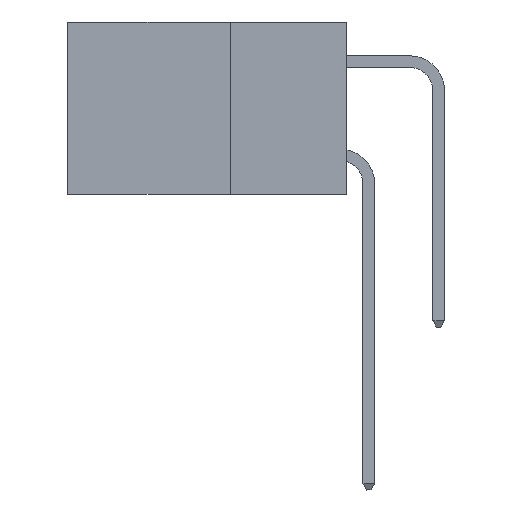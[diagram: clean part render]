
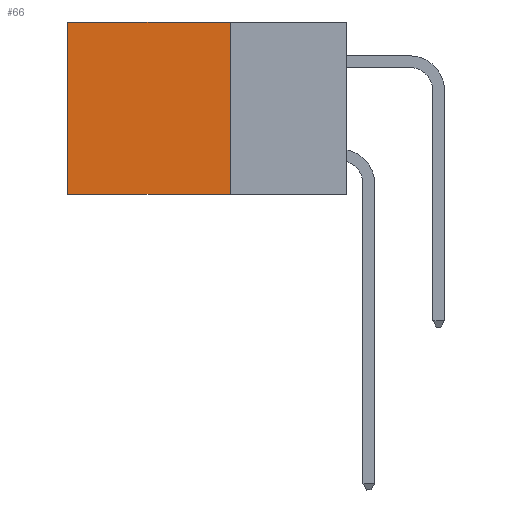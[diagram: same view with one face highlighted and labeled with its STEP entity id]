
A CAD part, left-side view. The second image highlights one B-rep face of the part: STEP entity #66.
In plain terms, the highlighted planar face has unit normal (-1, 0, 0).
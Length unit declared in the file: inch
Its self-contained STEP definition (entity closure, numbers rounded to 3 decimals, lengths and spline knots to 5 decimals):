
#66 = ADVANCED_FACE ( 'NONE', ( #22812 ), #25217, .F. ) ;
#1193 = ORIENTED_EDGE ( 'NONE', *, *, #30866, .T. ) ;
#2243 = CARTESIAN_POINT ( 'NONE',  ( 0.2875, 0.6, -0.37 ) ) ;
#3347 = CARTESIAN_POINT ( 'NONE',  ( 0.2875, 0.25, 0. ) ) ;
#4271 = CARTESIAN_POINT ( 'NONE',  ( 0.2875, 0.6, 0. ) ) ;
#4309 = DIRECTION ( 'NONE',  ( 0., 1., 0. ) ) ;
#5776 = DIRECTION ( 'NONE',  ( 0., 0., -1. ) ) ;
#6058 = EDGE_CURVE ( 'NONE', #28198, #13046, #10988, .T. ) ;
#7293 = CARTESIAN_POINT ( 'NONE',  ( 0.2875, 0.25, 0. ) ) ;
#7605 = DIRECTION ( 'NONE',  ( 0., 1., 0. ) ) ;
#8965 = VECTOR ( 'NONE', #19105, 39.37008 ) ;
#9306 = LINE ( 'NONE', #14015, #28712 ) ;
#9942 = CARTESIAN_POINT ( 'NONE',  ( 0.2875, 0.25, -0.37 ) ) ;
#10559 = ORIENTED_EDGE ( 'NONE', *, *, #6058, .F. ) ;
#10988 = LINE ( 'NONE', #20766, #12527 ) ;
#12527 = VECTOR ( 'NONE', #23336, 39.37008 ) ;
#13046 = VERTEX_POINT ( 'NONE', #9942 ) ;
#13366 = AXIS2_PLACEMENT_3D ( 'NONE', #3347, #15956, #5776 ) ;
#14015 = CARTESIAN_POINT ( 'NONE',  ( 0.2875, 0.25, -0.37 ) ) ;
#15956 = DIRECTION ( 'NONE',  ( 1., 0., 0. ) ) ;
#17403 = CARTESIAN_POINT ( 'NONE',  ( 0.2875, 0.25, 0. ) ) ;
#17987 = ORIENTED_EDGE ( 'NONE', *, *, #26063, .F. ) ;
#18203 = CARTESIAN_POINT ( 'NONE',  ( 0.2875, 0.6, 0. ) ) ;
#18378 = VERTEX_POINT ( 'NONE', #2243 ) ;
#19105 = DIRECTION ( 'NONE',  ( 0., 0., -1. ) ) ;
#19309 = EDGE_CURVE ( 'NONE', #28295, #18378, #24211, .T. ) ;
#20766 = CARTESIAN_POINT ( 'NONE',  ( 0.2875, 0.25, 0. ) ) ;
#21919 = LINE ( 'NONE', #7293, #31662 ) ;
#22150 = EDGE_LOOP ( 'NONE', ( #31398, #17987, #10559, #1193 ) ) ;
#22812 = FACE_OUTER_BOUND ( 'NONE', #22150, .T. ) ;
#23336 = DIRECTION ( 'NONE',  ( 0., 0., -1. ) ) ;
#24211 = LINE ( 'NONE', #4271, #8965 ) ;
#25217 = PLANE ( 'NONE',  #13366 ) ;
#26063 = EDGE_CURVE ( 'NONE', #13046, #18378, #9306, .T. ) ;
#28198 = VERTEX_POINT ( 'NONE', #17403 ) ;
#28295 = VERTEX_POINT ( 'NONE', #18203 ) ;
#28712 = VECTOR ( 'NONE', #4309, 39.37008 ) ;
#30866 = EDGE_CURVE ( 'NONE', #28198, #28295, #21919, .T. ) ;
#31398 = ORIENTED_EDGE ( 'NONE', *, *, #19309, .T. ) ;
#31662 = VECTOR ( 'NONE', #7605, 39.37008 ) ;
